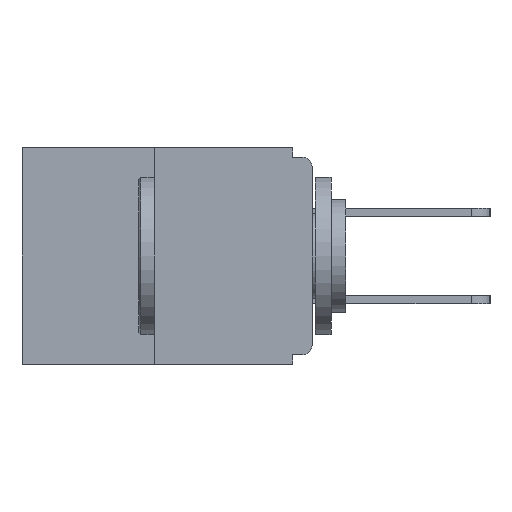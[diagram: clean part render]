
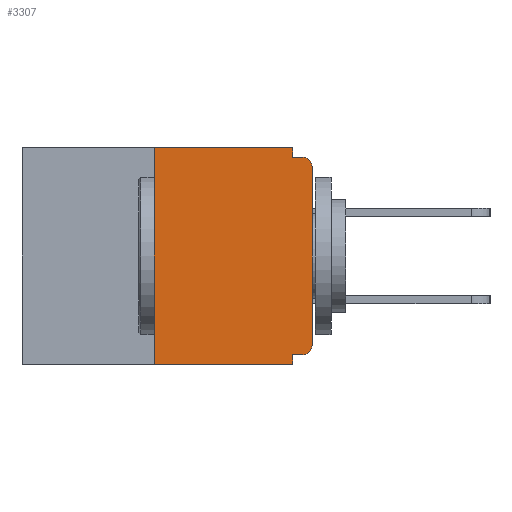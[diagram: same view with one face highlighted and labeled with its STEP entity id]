
A CAD part, left-side view. The second image highlights one B-rep face of the part: STEP entity #3307.
In plain terms, the highlighted planar face has unit normal (-1, 0, 0).
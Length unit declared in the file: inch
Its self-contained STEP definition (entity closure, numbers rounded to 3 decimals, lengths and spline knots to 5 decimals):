
#779 = ORIENTED_EDGE ( 'NONE', *, *, #19296, .F. ) ;
#868 = LINE ( 'NONE', #2724, #25689 ) ;
#1185 = CARTESIAN_POINT ( 'NONE',  ( 0., 0.46, -0.343 ) ) ;
#1306 = VERTEX_POINT ( 'NONE', #19472 ) ;
#2534 = PLANE ( 'NONE',  #4664 ) ;
#2724 = CARTESIAN_POINT ( 'NONE',  ( 0., 0.031, 0. ) ) ;
#2990 = DIRECTION ( 'NONE',  ( 0., -1., 0. ) ) ;
#3219 = VERTEX_POINT ( 'NONE', #18470 ) ;
#3307 = ADVANCED_FACE ( 'NONE', ( #13677 ), #2534, .F. ) ;
#3650 = CIRCLE ( 'NONE', #15635, 0.015 ) ;
#4190 = VECTOR ( 'NONE', #8460, 39.37008 ) ;
#4561 = VERTEX_POINT ( 'NONE', #19612 ) ;
#4664 = AXIS2_PLACEMENT_3D ( 'NONE', #4855, #22911, #16837 ) ;
#4826 = ORIENTED_EDGE ( 'NONE', *, *, #10895, .T. ) ;
#4855 = CARTESIAN_POINT ( 'NONE',  ( 0., 0.46, 0. ) ) ;
#4925 = ORIENTED_EDGE ( 'NONE', *, *, #7152, .F. ) ;
#5041 = CARTESIAN_POINT ( 'NONE',  ( 0., 0.031, -0.343 ) ) ;
#5163 = DIRECTION ( 'NONE',  ( -1., 0., 0. ) ) ;
#5181 = CARTESIAN_POINT ( 'NONE',  ( 0., 0., -0.03 ) ) ;
#6010 = EDGE_CURVE ( 'NONE', #4561, #14464, #15448, .T. ) ;
#6525 = ORIENTED_EDGE ( 'NONE', *, *, #8143, .T. ) ;
#6912 = DIRECTION ( 'NONE',  ( 0., 0., 1. ) ) ;
#7152 = EDGE_CURVE ( 'NONE', #14950, #3219, #22101, .T. ) ;
#7371 = LINE ( 'NONE', #10302, #4190 ) ;
#7514 = DIRECTION ( 'NONE',  ( 0., 0., -1. ) ) ;
#8143 = EDGE_CURVE ( 'NONE', #13976, #20977, #9021, .T. ) ;
#8460 = DIRECTION ( 'NONE',  ( 0., -1., 0. ) ) ;
#8669 = EDGE_CURVE ( 'NONE', #13976, #14950, #21300, .T. ) ;
#9021 = LINE ( 'NONE', #1185, #14713 ) ;
#9547 = LINE ( 'NONE', #12867, #24500 ) ;
#10033 = VECTOR ( 'NONE', #10108, 39.37008 ) ;
#10108 = DIRECTION ( 'NONE',  ( 0., 1., 0. ) ) ;
#10240 = ORIENTED_EDGE ( 'NONE', *, *, #13513, .T. ) ;
#10248 = CARTESIAN_POINT ( 'NONE',  ( 0., 0.25, -0.343 ) ) ;
#10302 = CARTESIAN_POINT ( 'NONE',  ( 0., 0., -0.015 ) ) ;
#10562 = EDGE_CURVE ( 'NONE', #14464, #20977, #23429, .T. ) ;
#10895 = EDGE_CURVE ( 'NONE', #24581, #1306, #3650, .T. ) ;
#12831 = EDGE_CURVE ( 'NONE', #25516, #1306, #7371, .T. ) ;
#12867 = CARTESIAN_POINT ( 'NONE',  ( 0., 0., 0. ) ) ;
#12929 = CARTESIAN_POINT ( 'NONE',  ( 0., 0.031, -0.015 ) ) ;
#13513 = EDGE_CURVE ( 'NONE', #22373, #24581, #9547, .T. ) ;
#13677 = FACE_OUTER_BOUND ( 'NONE', #15676, .T. ) ;
#13976 = VERTEX_POINT ( 'NONE', #10248 ) ;
#14427 = CARTESIAN_POINT ( 'NONE',  ( 0., 0.031, -0.343 ) ) ;
#14464 = VERTEX_POINT ( 'NONE', #20054 ) ;
#14713 = VECTOR ( 'NONE', #19169, 39.37008 ) ;
#14950 = VERTEX_POINT ( 'NONE', #18121 ) ;
#15448 = LINE ( 'NONE', #26260, #10033 ) ;
#15635 = AXIS2_PLACEMENT_3D ( 'NONE', #17117, #20004, #7514 ) ;
#15676 = EDGE_LOOP ( 'NONE', ( #4925, #21345, #6525, #16635, #24461, #24815, #10240, #4826, #20779, #779 ) ) ;
#16053 = EDGE_CURVE ( 'NONE', #4561, #22373, #17530, .T. ) ;
#16635 = ORIENTED_EDGE ( 'NONE', *, *, #10562, .F. ) ;
#16836 = CARTESIAN_POINT ( 'NONE',  ( 0., 0., -0.313 ) ) ;
#16837 = DIRECTION ( 'NONE',  ( 0., 0., -1. ) ) ;
#17117 = CARTESIAN_POINT ( 'NONE',  ( 0., 0.015, -0.03 ) ) ;
#17246 = CARTESIAN_POINT ( 'NONE',  ( 0., 0.25, 0. ) ) ;
#17348 = CARTESIAN_POINT ( 'NONE',  ( 0., 0.015, -0.313 ) ) ;
#17530 = CIRCLE ( 'NONE', #18990, 0.015 ) ;
#17992 = VECTOR ( 'NONE', #22546, 39.37008 ) ;
#18121 = CARTESIAN_POINT ( 'NONE',  ( 0., 0.25, 0. ) ) ;
#18470 = CARTESIAN_POINT ( 'NONE',  ( 0., 0.031, 0. ) ) ;
#18990 = AXIS2_PLACEMENT_3D ( 'NONE', #17348, #5163, #25543 ) ;
#19169 = DIRECTION ( 'NONE',  ( 0., -1., 0. ) ) ;
#19296 = EDGE_CURVE ( 'NONE', #3219, #25516, #868, .T. ) ;
#19472 = CARTESIAN_POINT ( 'NONE',  ( 0., 0.015, -0.015 ) ) ;
#19612 = CARTESIAN_POINT ( 'NONE',  ( 0., 0.015, -0.328 ) ) ;
#20004 = DIRECTION ( 'NONE',  ( -1., 0., 0. ) ) ;
#20016 = VECTOR ( 'NONE', #23561, 39.37008 ) ;
#20054 = CARTESIAN_POINT ( 'NONE',  ( 0., 0.031, -0.328 ) ) ;
#20779 = ORIENTED_EDGE ( 'NONE', *, *, #12831, .F. ) ;
#20893 = CARTESIAN_POINT ( 'NONE',  ( 0., 0.46, 0. ) ) ;
#20977 = VERTEX_POINT ( 'NONE', #5041 ) ;
#21300 = LINE ( 'NONE', #17246, #20016 ) ;
#21345 = ORIENTED_EDGE ( 'NONE', *, *, #8669, .F. ) ;
#22101 = LINE ( 'NONE', #20893, #23399 ) ;
#22373 = VERTEX_POINT ( 'NONE', #16836 ) ;
#22546 = DIRECTION ( 'NONE',  ( 0., 0., -1. ) ) ;
#22911 = DIRECTION ( 'NONE',  ( 1., 0., 0. ) ) ;
#23399 = VECTOR ( 'NONE', #2990, 39.37008 ) ;
#23429 = LINE ( 'NONE', #14427, #17992 ) ;
#23561 = DIRECTION ( 'NONE',  ( 0., 0., 1. ) ) ;
#24461 = ORIENTED_EDGE ( 'NONE', *, *, #6010, .F. ) ;
#24500 = VECTOR ( 'NONE', #6912, 39.37008 ) ;
#24581 = VERTEX_POINT ( 'NONE', #5181 ) ;
#24776 = DIRECTION ( 'NONE',  ( 0., 0., -1. ) ) ;
#24815 = ORIENTED_EDGE ( 'NONE', *, *, #16053, .T. ) ;
#25516 = VERTEX_POINT ( 'NONE', #12929 ) ;
#25543 = DIRECTION ( 'NONE',  ( 0., 0., -1. ) ) ;
#25689 = VECTOR ( 'NONE', #24776, 39.37008 ) ;
#26260 = CARTESIAN_POINT ( 'NONE',  ( 0., 0., -0.328 ) ) ;
